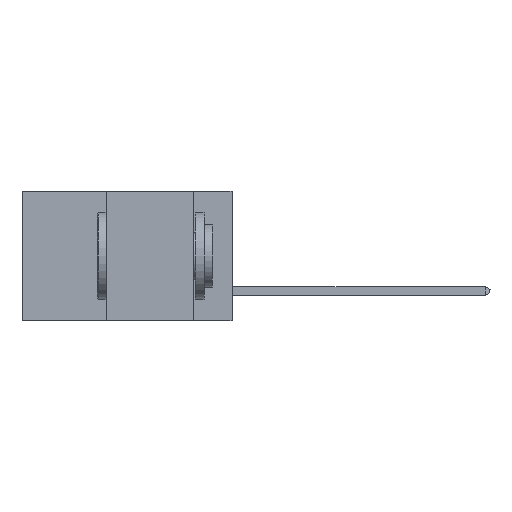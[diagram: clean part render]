
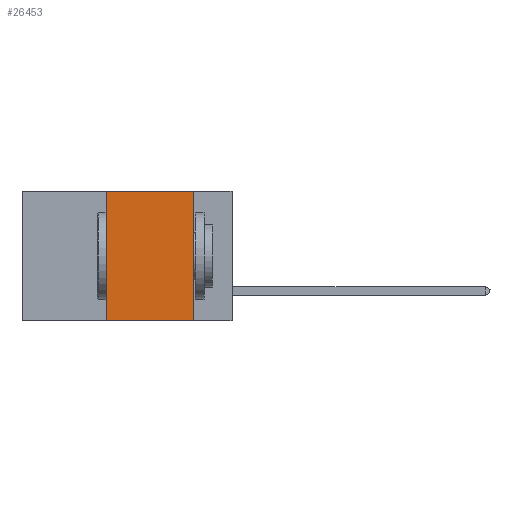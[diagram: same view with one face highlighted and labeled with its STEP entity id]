
A CAD part, left-side view. The second image highlights one B-rep face of the part: STEP entity #26453.
In plain terms, the highlighted planar face has unit normal (-1, 0, 0).
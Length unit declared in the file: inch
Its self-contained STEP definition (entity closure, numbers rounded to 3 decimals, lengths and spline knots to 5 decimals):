
#2230 = ORIENTED_EDGE ( 'NONE', *, *, #41470, .F. ) ;
#3037 = ORIENTED_EDGE ( 'NONE', *, *, #3821, .F. ) ;
#3821 = EDGE_CURVE ( 'NONE', #31219, #24540, #21134, .T. ) ;
#3922 = VERTEX_POINT ( 'NONE', #9232 ) ;
#4203 = DIRECTION ( 'NONE',  ( 0., -1., 0. ) ) ;
#4874 = CARTESIAN_POINT ( 'NONE',  ( 0., 0.36, 0. ) ) ;
#5477 = CARTESIAN_POINT ( 'NONE',  ( 0., 0.6, -0.37 ) ) ;
#6408 = CARTESIAN_POINT ( 'NONE',  ( 0., 0.11, -0.37 ) ) ;
#6447 = DIRECTION ( 'NONE',  ( 0., 0., -1. ) ) ;
#6753 = DIRECTION ( 'NONE',  ( 1., 0., 0. ) ) ;
#7063 = EDGE_CURVE ( 'NONE', #3922, #25693, #22740, .T. ) ;
#7339 = CARTESIAN_POINT ( 'NONE',  ( 0., 0.36, 0. ) ) ;
#7420 = AXIS2_PLACEMENT_3D ( 'NONE', #12821, #6753, #6447 ) ;
#9232 = CARTESIAN_POINT ( 'NONE',  ( 0., 0.36, -0.37 ) ) ;
#10440 = ORIENTED_EDGE ( 'NONE', *, *, #27750, .F. ) ;
#12821 = CARTESIAN_POINT ( 'NONE',  ( 0., 0.6, 0. ) ) ;
#16623 = PLANE ( 'NONE',  #7420 ) ;
#17629 = VECTOR ( 'NONE', #27752, 39.37008 ) ;
#17932 = VECTOR ( 'NONE', #21982, 39.37008 ) ;
#18151 = EDGE_LOOP ( 'NONE', ( #10440, #3037, #2230, #20047 ) ) ;
#20047 = ORIENTED_EDGE ( 'NONE', *, *, #7063, .T. ) ;
#21134 = LINE ( 'NONE', #22214, #40949 ) ;
#21443 = CARTESIAN_POINT ( 'NONE',  ( 0., 0.11, 0. ) ) ;
#21982 = DIRECTION ( 'NONE',  ( 0., 0., -1. ) ) ;
#22214 = CARTESIAN_POINT ( 'NONE',  ( 0., 0.6, 0. ) ) ;
#22740 = LINE ( 'NONE', #5477, #17629 ) ;
#24540 = VERTEX_POINT ( 'NONE', #21443 ) ;
#25626 = DIRECTION ( 'NONE',  ( 0., 0., 1. ) ) ;
#25693 = VERTEX_POINT ( 'NONE', #6408 ) ;
#26453 = ADVANCED_FACE ( 'NONE', ( #36178 ), #16623, .F. ) ;
#27634 = LINE ( 'NONE', #34203, #17932 ) ;
#27750 = EDGE_CURVE ( 'NONE', #24540, #25693, #27634, .T. ) ;
#27752 = DIRECTION ( 'NONE',  ( 0., -1., 0. ) ) ;
#31219 = VERTEX_POINT ( 'NONE', #4874 ) ;
#31817 = VECTOR ( 'NONE', #25626, 39.37008 ) ;
#34203 = CARTESIAN_POINT ( 'NONE',  ( 0., 0.11, 0. ) ) ;
#36178 = FACE_OUTER_BOUND ( 'NONE', #18151, .T. ) ;
#40949 = VECTOR ( 'NONE', #4203, 39.37008 ) ;
#41470 = EDGE_CURVE ( 'NONE', #3922, #31219, #42551, .T. ) ;
#42551 = LINE ( 'NONE', #7339, #31817 ) ;
